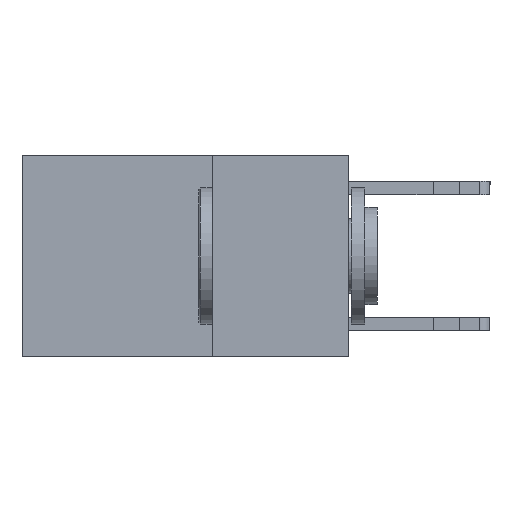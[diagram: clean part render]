
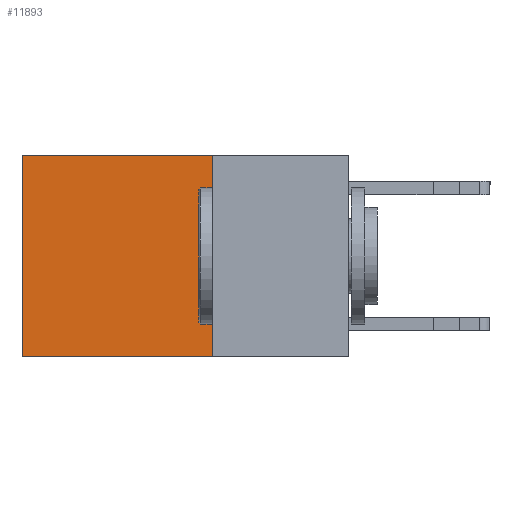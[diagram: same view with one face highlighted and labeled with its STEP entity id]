
A CAD part, left-side view. The second image highlights one B-rep face of the part: STEP entity #11893.
In plain terms, the highlighted planar face has unit normal (-1, 0, 0).
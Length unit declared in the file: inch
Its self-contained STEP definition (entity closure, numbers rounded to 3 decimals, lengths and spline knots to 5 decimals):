
#110 = CARTESIAN_POINT ( 'NONE',  ( 0.2625, 0.25, 0. ) ) ;
#578 = VECTOR ( 'NONE', #7805, 39.37008 ) ;
#687 = EDGE_CURVE ( 'NONE', #6968, #11054, #3324, .T. ) ;
#759 = LINE ( 'NONE', #5425, #3272 ) ;
#1113 = EDGE_LOOP ( 'NONE', ( #11671, #9406, #6678, #4115 ) ) ;
#1267 = VERTEX_POINT ( 'NONE', #13632 ) ;
#1721 = EDGE_CURVE ( 'NONE', #1267, #12925, #1989, .T. ) ;
#1816 = EDGE_CURVE ( 'NONE', #1267, #6968, #759, .T. ) ;
#1989 = LINE ( 'NONE', #11392, #578 ) ;
#2277 = CARTESIAN_POINT ( 'NONE',  ( 0.2625, 0.6, 0. ) ) ;
#3215 = AXIS2_PLACEMENT_3D ( 'NONE', #110, #6926, #5695 ) ;
#3272 = VECTOR ( 'NONE', #8954, 39.37008 ) ;
#3324 = LINE ( 'NONE', #6846, #4045 ) ;
#3422 = DIRECTION ( 'NONE',  ( 0., 0., -1. ) ) ;
#4045 = VECTOR ( 'NONE', #14852, 39.37008 ) ;
#4115 = ORIENTED_EDGE ( 'NONE', *, *, #1721, .T. ) ;
#5231 = EDGE_CURVE ( 'NONE', #12925, #11054, #6875, .T. ) ;
#5425 = CARTESIAN_POINT ( 'NONE',  ( 0.2625, 0.25, 0. ) ) ;
#5695 = DIRECTION ( 'NONE',  ( 0., 0., -1. ) ) ;
#6678 = ORIENTED_EDGE ( 'NONE', *, *, #1816, .F. ) ;
#6722 = CARTESIAN_POINT ( 'NONE',  ( 0.2625, 0.25, -0.37 ) ) ;
#6846 = CARTESIAN_POINT ( 'NONE',  ( 0.2625, 0.25, -0.37 ) ) ;
#6875 = LINE ( 'NONE', #2277, #12383 ) ;
#6926 = DIRECTION ( 'NONE',  ( 1., 0., 0. ) ) ;
#6968 = VERTEX_POINT ( 'NONE', #6722 ) ;
#7219 = PLANE ( 'NONE',  #3215 ) ;
#7696 = CARTESIAN_POINT ( 'NONE',  ( 0.2625, 0.6, 0. ) ) ;
#7805 = DIRECTION ( 'NONE',  ( 0., 1., 0. ) ) ;
#8954 = DIRECTION ( 'NONE',  ( 0., 0., -1. ) ) ;
#9406 = ORIENTED_EDGE ( 'NONE', *, *, #687, .F. ) ;
#9525 = FACE_OUTER_BOUND ( 'NONE', #1113, .T. ) ;
#11054 = VERTEX_POINT ( 'NONE', #11702 ) ;
#11392 = CARTESIAN_POINT ( 'NONE',  ( 0.2625, 0.25, 0. ) ) ;
#11671 = ORIENTED_EDGE ( 'NONE', *, *, #5231, .T. ) ;
#11702 = CARTESIAN_POINT ( 'NONE',  ( 0.2625, 0.6, -0.37 ) ) ;
#11893 = ADVANCED_FACE ( 'NONE', ( #9525 ), #7219, .F. ) ;
#12383 = VECTOR ( 'NONE', #3422, 39.37008 ) ;
#12925 = VERTEX_POINT ( 'NONE', #7696 ) ;
#13632 = CARTESIAN_POINT ( 'NONE',  ( 0.2625, 0.25, 0. ) ) ;
#14852 = DIRECTION ( 'NONE',  ( 0., 1., 0. ) ) ;
